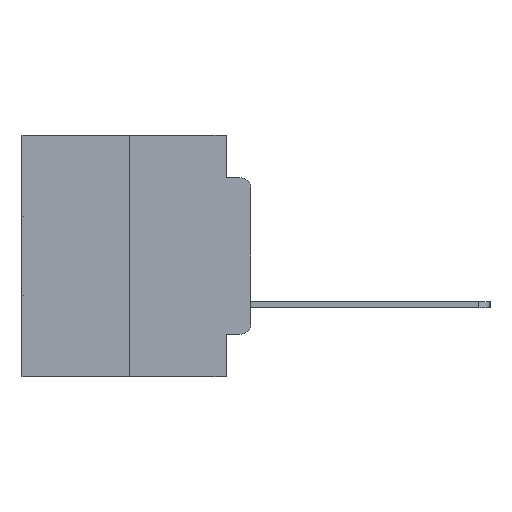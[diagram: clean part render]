
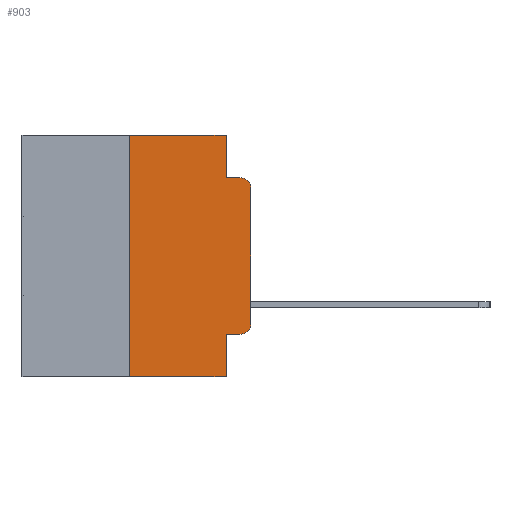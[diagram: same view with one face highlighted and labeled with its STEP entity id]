
A CAD part, left-side view. The second image highlights one B-rep face of the part: STEP entity #903.
In plain terms, the highlighted planar face has unit normal (-1, 0, 0).
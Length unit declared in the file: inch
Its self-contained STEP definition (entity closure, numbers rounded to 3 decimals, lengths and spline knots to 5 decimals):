
#849 = ORIENTED_EDGE ( 'NONE', *, *, #24464, .T. ) ;
#903 = ADVANCED_FACE ( 'NONE', ( #19062 ), #24875, .F. ) ;
#1271 = CARTESIAN_POINT ( 'NONE',  ( 0., 0.051, 0. ) ) ;
#1465 = EDGE_CURVE ( 'NONE', #9003, #21508, #4699, .T. ) ;
#1719 = VERTEX_POINT ( 'NONE', #29928 ) ;
#2032 = VERTEX_POINT ( 'NONE', #12792 ) ;
#2158 = CARTESIAN_POINT ( 'NONE',  ( 0., 0.051, -0.0885 ) ) ;
#2344 = LINE ( 'NONE', #22564, #25846 ) ;
#2670 = CARTESIAN_POINT ( 'NONE',  ( 0., 0.051, 0. ) ) ;
#2822 = EDGE_CURVE ( 'NONE', #9294, #9003, #7856, .T. ) ;
#2846 = DIRECTION ( 'NONE',  ( 0., 0., -1. ) ) ;
#3587 = VERTEX_POINT ( 'NONE', #27460 ) ;
#4278 = ORIENTED_EDGE ( 'NONE', *, *, #12750, .T. ) ;
#4656 = EDGE_LOOP ( 'NONE', ( #16436, #4278, #22184, #12808, #17959, #11719, #29199, #12421, #849, #21143 ) ) ;
#4699 = LINE ( 'NONE', #9542, #28900 ) ;
#5540 = EDGE_CURVE ( 'NONE', #21508, #11805, #19195, .T. ) ;
#5944 = VECTOR ( 'NONE', #23168, 39.37008 ) ;
#6575 = VERTEX_POINT ( 'NONE', #28089 ) ;
#6878 = CARTESIAN_POINT ( 'NONE',  ( 0., 0.473, -0.5 ) ) ;
#7258 = VECTOR ( 'NONE', #18570, 39.37008 ) ;
#7744 = CARTESIAN_POINT ( 'NONE',  ( 0., 0.25, 0. ) ) ;
#7784 = DIRECTION ( 'NONE',  ( -1., 0., 0. ) ) ;
#7805 = CARTESIAN_POINT ( 'NONE',  ( 0., 0.02, -0.3915 ) ) ;
#7856 = LINE ( 'NONE', #23473, #15029 ) ;
#7984 = VECTOR ( 'NONE', #13679, 39.37008 ) ;
#8484 = EDGE_CURVE ( 'NONE', #9294, #11571, #23876, .T. ) ;
#9003 = VERTEX_POINT ( 'NONE', #7744 ) ;
#9294 = VERTEX_POINT ( 'NONE', #16318 ) ;
#9542 = CARTESIAN_POINT ( 'NONE',  ( 0., 0.473, 0. ) ) ;
#9760 = AXIS2_PLACEMENT_3D ( 'NONE', #21902, #7784, #24016 ) ;
#10342 = DIRECTION ( 'NONE',  ( 0., 0., -1. ) ) ;
#10441 = AXIS2_PLACEMENT_3D ( 'NONE', #21952, #29611, #2846 ) ;
#11086 = DIRECTION ( 'NONE',  ( 0., 0., 1. ) ) ;
#11264 = EDGE_CURVE ( 'NONE', #1719, #21144, #2344, .T. ) ;
#11571 = VERTEX_POINT ( 'NONE', #22989 ) ;
#11719 = ORIENTED_EDGE ( 'NONE', *, *, #2822, .F. ) ;
#11805 = VERTEX_POINT ( 'NONE', #2158 ) ;
#12069 = CIRCLE ( 'NONE', #12523, 0.02 ) ;
#12421 = ORIENTED_EDGE ( 'NONE', *, *, #15493, .F. ) ;
#12523 = AXIS2_PLACEMENT_3D ( 'NONE', #7805, #24034, #10342 ) ;
#12750 = EDGE_CURVE ( 'NONE', #21144, #3587, #22245, .T. ) ;
#12792 = CARTESIAN_POINT ( 'NONE',  ( 0., 0.051, -0.4115 ) ) ;
#12808 = ORIENTED_EDGE ( 'NONE', *, *, #5540, .F. ) ;
#13679 = DIRECTION ( 'NONE',  ( 0., -1., 0. ) ) ;
#14049 = DIRECTION ( 'NONE',  ( 0., -1., 0. ) ) ;
#15029 = VECTOR ( 'NONE', #23456, 39.37008 ) ;
#15493 = EDGE_CURVE ( 'NONE', #2032, #11571, #25097, .T. ) ;
#15708 = CARTESIAN_POINT ( 'NONE',  ( 0., 0., -0.1085 ) ) ;
#15807 = CARTESIAN_POINT ( 'NONE',  ( 0., 0.051, -0.4115 ) ) ;
#15883 = VECTOR ( 'NONE', #20468, 39.37008 ) ;
#16318 = CARTESIAN_POINT ( 'NONE',  ( 0., 0.25, -0.5 ) ) ;
#16436 = ORIENTED_EDGE ( 'NONE', *, *, #11264, .T. ) ;
#17959 = ORIENTED_EDGE ( 'NONE', *, *, #1465, .F. ) ;
#18570 = DIRECTION ( 'NONE',  ( 0., 0., -1. ) ) ;
#19062 = FACE_OUTER_BOUND ( 'NONE', #4656, .T. ) ;
#19195 = LINE ( 'NONE', #1271, #7258 ) ;
#19397 = VECTOR ( 'NONE', #23942, 39.37008 ) ;
#20468 = DIRECTION ( 'NONE',  ( 0., -1., 0. ) ) ;
#20580 = LINE ( 'NONE', #26874, #7984 ) ;
#21143 = ORIENTED_EDGE ( 'NONE', *, *, #27195, .T. ) ;
#21144 = VERTEX_POINT ( 'NONE', #15708 ) ;
#21508 = VERTEX_POINT ( 'NONE', #27764 ) ;
#21902 = CARTESIAN_POINT ( 'NONE',  ( 0., 0.02, -0.1085 ) ) ;
#21952 = CARTESIAN_POINT ( 'NONE',  ( 0., 0.473, 0. ) ) ;
#21985 = LINE ( 'NONE', #15807, #15883 ) ;
#22184 = ORIENTED_EDGE ( 'NONE', *, *, #24543, .F. ) ;
#22245 = CIRCLE ( 'NONE', #9760, 0.02 ) ;
#22564 = CARTESIAN_POINT ( 'NONE',  ( 0., 0., 0. ) ) ;
#22989 = CARTESIAN_POINT ( 'NONE',  ( 0., 0.051, -0.5 ) ) ;
#23168 = DIRECTION ( 'NONE',  ( 0., -1., 0. ) ) ;
#23456 = DIRECTION ( 'NONE',  ( 0., 0., 1. ) ) ;
#23473 = CARTESIAN_POINT ( 'NONE',  ( 0., 0.25, 0. ) ) ;
#23876 = LINE ( 'NONE', #6878, #5944 ) ;
#23942 = DIRECTION ( 'NONE',  ( 0., 0., -1. ) ) ;
#24016 = DIRECTION ( 'NONE',  ( 0., 0., -1. ) ) ;
#24034 = DIRECTION ( 'NONE',  ( -1., 0., 0. ) ) ;
#24464 = EDGE_CURVE ( 'NONE', #2032, #6575, #21985, .T. ) ;
#24543 = EDGE_CURVE ( 'NONE', #11805, #3587, #20580, .T. ) ;
#24875 = PLANE ( 'NONE',  #10441 ) ;
#25097 = LINE ( 'NONE', #2670, #19397 ) ;
#25846 = VECTOR ( 'NONE', #11086, 39.37008 ) ;
#26874 = CARTESIAN_POINT ( 'NONE',  ( 0., 0.051, -0.0885 ) ) ;
#27195 = EDGE_CURVE ( 'NONE', #6575, #1719, #12069, .T. ) ;
#27460 = CARTESIAN_POINT ( 'NONE',  ( 0., 0.02, -0.0885 ) ) ;
#27764 = CARTESIAN_POINT ( 'NONE',  ( 0., 0.051, 0. ) ) ;
#28089 = CARTESIAN_POINT ( 'NONE',  ( 0., 0.02, -0.4115 ) ) ;
#28900 = VECTOR ( 'NONE', #14049, 39.37008 ) ;
#29199 = ORIENTED_EDGE ( 'NONE', *, *, #8484, .T. ) ;
#29611 = DIRECTION ( 'NONE',  ( 1., 0., 0. ) ) ;
#29928 = CARTESIAN_POINT ( 'NONE',  ( 0., 0., -0.3915 ) ) ;
